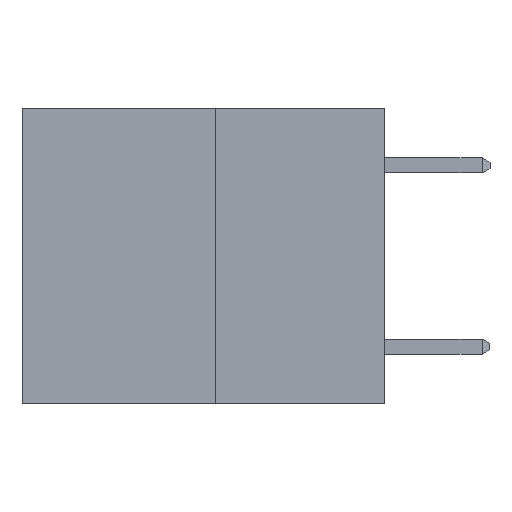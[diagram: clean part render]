
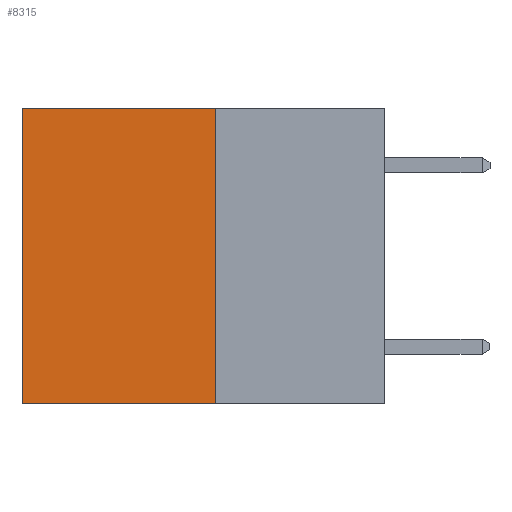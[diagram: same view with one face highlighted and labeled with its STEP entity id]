
A CAD part, left-side view. The second image highlights one B-rep face of the part: STEP entity #8315.
In plain terms, the highlighted planar face has unit normal (-1, 0, 0).
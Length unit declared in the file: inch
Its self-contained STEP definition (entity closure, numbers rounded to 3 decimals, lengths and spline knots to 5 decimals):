
#310 = EDGE_CURVE ( 'NONE', #6617, #10374, #3692, .T. ) ;
#461 = DIRECTION ( 'NONE',  ( 0., 1., 0. ) ) ;
#516 = CARTESIAN_POINT ( 'NONE',  ( 0.3165, 0.6, -0.49 ) ) ;
#520 = LINE ( 'NONE', #3392, #12799 ) ;
#904 = PLANE ( 'NONE',  #1408 ) ;
#1408 = AXIS2_PLACEMENT_3D ( 'NONE', #10022, #4867, #8053 ) ;
#1450 = EDGE_CURVE ( 'NONE', #6617, #9052, #7212, .T. ) ;
#1688 = CARTESIAN_POINT ( 'NONE',  ( 0.3165, 0.28, -0.49 ) ) ;
#2846 = CARTESIAN_POINT ( 'NONE',  ( 0.3165, 0.28, 0. ) ) ;
#3353 = DIRECTION ( 'NONE',  ( 0., 0., -1. ) ) ;
#3355 = VERTEX_POINT ( 'NONE', #516 ) ;
#3392 = CARTESIAN_POINT ( 'NONE',  ( 0.3165, 0.6, -0.49 ) ) ;
#3692 = LINE ( 'NONE', #9766, #11085 ) ;
#4867 = DIRECTION ( 'NONE',  ( 1., 0., 0. ) ) ;
#6551 = VECTOR ( 'NONE', #461, 39.37008 ) ;
#6617 = VERTEX_POINT ( 'NONE', #2846 ) ;
#7212 = LINE ( 'NONE', #7481, #6551 ) ;
#7481 = CARTESIAN_POINT ( 'NONE',  ( 0.3165, 0.28, 0. ) ) ;
#7581 = FACE_OUTER_BOUND ( 'NONE', #8405, .T. ) ;
#7603 = ORIENTED_EDGE ( 'NONE', *, *, #10999, .T. ) ;
#7827 = ORIENTED_EDGE ( 'NONE', *, *, #8955, .F. ) ;
#8053 = DIRECTION ( 'NONE',  ( 0., 0., -1. ) ) ;
#8315 = ADVANCED_FACE ( 'NONE', ( #7581 ), #904, .F. ) ;
#8405 = EDGE_LOOP ( 'NONE', ( #7603, #7827, #12929, #11784 ) ) ;
#8955 = EDGE_CURVE ( 'NONE', #10374, #3355, #10445, .T. ) ;
#9052 = VERTEX_POINT ( 'NONE', #11197 ) ;
#9766 = CARTESIAN_POINT ( 'NONE',  ( 0.3165, 0.28, -0.49 ) ) ;
#9835 = DIRECTION ( 'NONE',  ( 0., 1., 0. ) ) ;
#10022 = CARTESIAN_POINT ( 'NONE',  ( 0.3165, 0.28, -0.49 ) ) ;
#10374 = VERTEX_POINT ( 'NONE', #11725 ) ;
#10445 = LINE ( 'NONE', #1688, #11400 ) ;
#10999 = EDGE_CURVE ( 'NONE', #9052, #3355, #520, .T. ) ;
#11085 = VECTOR ( 'NONE', #12864, 39.37008 ) ;
#11197 = CARTESIAN_POINT ( 'NONE',  ( 0.3165, 0.6, 0. ) ) ;
#11400 = VECTOR ( 'NONE', #9835, 39.37008 ) ;
#11725 = CARTESIAN_POINT ( 'NONE',  ( 0.3165, 0.28, -0.49 ) ) ;
#11784 = ORIENTED_EDGE ( 'NONE', *, *, #1450, .T. ) ;
#12799 = VECTOR ( 'NONE', #3353, 39.37008 ) ;
#12864 = DIRECTION ( 'NONE',  ( 0., 0., -1. ) ) ;
#12929 = ORIENTED_EDGE ( 'NONE', *, *, #310, .F. ) ;
